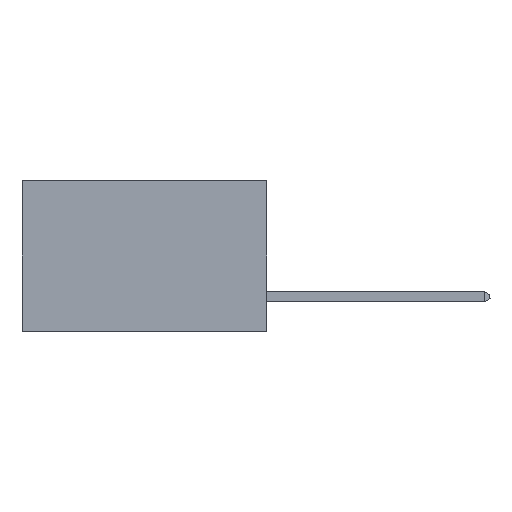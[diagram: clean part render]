
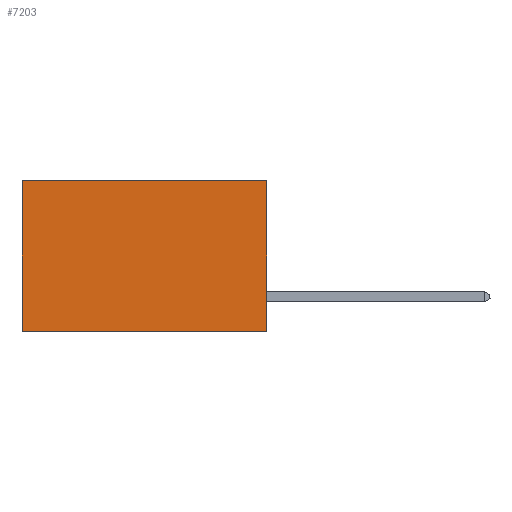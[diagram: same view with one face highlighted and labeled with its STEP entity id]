
A CAD part, left-side view. The second image highlights one B-rep face of the part: STEP entity #7203.
In plain terms, the highlighted planar face has unit normal (-1, 0, 0).
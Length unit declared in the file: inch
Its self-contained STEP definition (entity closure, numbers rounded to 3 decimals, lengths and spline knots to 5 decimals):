
#2618 = PLANE ( 'NONE',  #5794 ) ;
#3564 = CARTESIAN_POINT ( 'NONE',  ( 0.2875, 0., 0. ) ) ;
#5322 = FACE_OUTER_BOUND ( 'NONE', #27124, .T. ) ;
#5615 = CARTESIAN_POINT ( 'NONE',  ( 0.2875, 0.6, -0.37 ) ) ;
#5794 = AXIS2_PLACEMENT_3D ( 'NONE', #20217, #10364, #15522 ) ;
#6699 = EDGE_CURVE ( 'NONE', #16925, #29097, #25823, .T. ) ;
#6931 = VECTOR ( 'NONE', #12347, 39.37008 ) ;
#7029 = DIRECTION ( 'NONE',  ( 0., 0., -1. ) ) ;
#7203 = ADVANCED_FACE ( 'NONE', ( #5322 ), #2618, .F. ) ;
#7330 = DIRECTION ( 'NONE',  ( 0., 0., -1. ) ) ;
#8092 = EDGE_CURVE ( 'NONE', #11119, #32245, #20981, .T. ) ;
#8607 = ORIENTED_EDGE ( 'NONE', *, *, #6699, .T. ) ;
#10364 = DIRECTION ( 'NONE',  ( 1., 0., 0. ) ) ;
#11119 = VERTEX_POINT ( 'NONE', #21353 ) ;
#12347 = DIRECTION ( 'NONE',  ( 0., 1., 0. ) ) ;
#12831 = VECTOR ( 'NONE', #7029, 39.37008 ) ;
#14688 = ORIENTED_EDGE ( 'NONE', *, *, #14877, .T. ) ;
#14877 = EDGE_CURVE ( 'NONE', #29097, #32245, #16769, .T. ) ;
#15522 = DIRECTION ( 'NONE',  ( 0., 0., -1. ) ) ;
#16230 = CARTESIAN_POINT ( 'NONE',  ( 0.2875, 0.6, 0. ) ) ;
#16769 = LINE ( 'NONE', #25098, #20717 ) ;
#16925 = VERTEX_POINT ( 'NONE', #3564 ) ;
#18181 = DIRECTION ( 'NONE',  ( 0., 1., 0. ) ) ;
#18689 = LINE ( 'NONE', #22041, #12831 ) ;
#19547 = CARTESIAN_POINT ( 'NONE',  ( 0.2875, 0., 0. ) ) ;
#20217 = CARTESIAN_POINT ( 'NONE',  ( 0.2875, 0., 0. ) ) ;
#20717 = VECTOR ( 'NONE', #7330, 39.37008 ) ;
#20981 = LINE ( 'NONE', #27974, #24091 ) ;
#21353 = CARTESIAN_POINT ( 'NONE',  ( 0.2875, 0., -0.37 ) ) ;
#21362 = ORIENTED_EDGE ( 'NONE', *, *, #8092, .F. ) ;
#22041 = CARTESIAN_POINT ( 'NONE',  ( 0.2875, 0., 0. ) ) ;
#22541 = ORIENTED_EDGE ( 'NONE', *, *, #24422, .F. ) ;
#24091 = VECTOR ( 'NONE', #18181, 39.37008 ) ;
#24422 = EDGE_CURVE ( 'NONE', #16925, #11119, #18689, .T. ) ;
#25098 = CARTESIAN_POINT ( 'NONE',  ( 0.2875, 0.6, 0. ) ) ;
#25823 = LINE ( 'NONE', #19547, #6931 ) ;
#27124 = EDGE_LOOP ( 'NONE', ( #14688, #21362, #22541, #8607 ) ) ;
#27974 = CARTESIAN_POINT ( 'NONE',  ( 0.2875, 0., -0.37 ) ) ;
#29097 = VERTEX_POINT ( 'NONE', #16230 ) ;
#32245 = VERTEX_POINT ( 'NONE', #5615 ) ;
